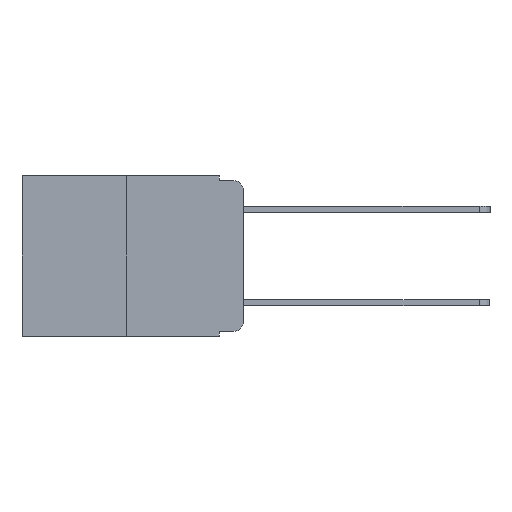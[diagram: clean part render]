
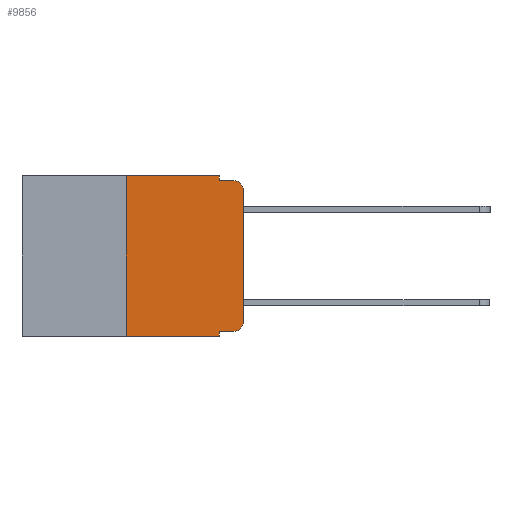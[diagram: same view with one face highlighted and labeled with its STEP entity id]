
A CAD part, left-side view. The second image highlights one B-rep face of the part: STEP entity #9856.
In plain terms, the highlighted planar face has unit normal (-1, 0, 0).
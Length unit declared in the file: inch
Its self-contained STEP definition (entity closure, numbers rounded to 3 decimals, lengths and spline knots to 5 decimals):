
#102 = CIRCLE ( 'NONE', #6710, 0.02 ) ;
#133 = DIRECTION ( 'NONE',  ( -1., 0., 0. ) ) ;
#184 = EDGE_CURVE ( 'NONE', #4571, #2796, #8095, .T. ) ;
#198 = VERTEX_POINT ( 'NONE', #6690 ) ;
#562 = DIRECTION ( 'NONE',  ( 0., -1., 0. ) ) ;
#798 = CARTESIAN_POINT ( 'NONE',  ( 0., 0.25, -0.343 ) ) ;
#813 = ORIENTED_EDGE ( 'NONE', *, *, #11226, .T. ) ;
#899 = VERTEX_POINT ( 'NONE', #11104 ) ;
#1318 = VECTOR ( 'NONE', #3321, 39.37008 ) ;
#1935 = CARTESIAN_POINT ( 'NONE',  ( 0., 0.473, 0. ) ) ;
#1977 = LINE ( 'NONE', #2537, #4477 ) ;
#2357 = CARTESIAN_POINT ( 'NONE',  ( 0., 0., 0. ) ) ;
#2383 = EDGE_CURVE ( 'NONE', #899, #3864, #1977, .T. ) ;
#2537 = CARTESIAN_POINT ( 'NONE',  ( 0., 0.051, -0.333 ) ) ;
#2681 = VERTEX_POINT ( 'NONE', #7798 ) ;
#2796 = VERTEX_POINT ( 'NONE', #7469 ) ;
#2858 = DIRECTION ( 'NONE',  ( 0., 0., -1. ) ) ;
#2948 = CARTESIAN_POINT ( 'NONE',  ( 0., 0.051, -0.343 ) ) ;
#3065 = VERTEX_POINT ( 'NONE', #4823 ) ;
#3231 = DIRECTION ( 'NONE',  ( 0., -1., 0. ) ) ;
#3321 = DIRECTION ( 'NONE',  ( 0., 0., 1. ) ) ;
#3358 = CARTESIAN_POINT ( 'NONE',  ( 0., 0., -0.03 ) ) ;
#3531 = ORIENTED_EDGE ( 'NONE', *, *, #9090, .T. ) ;
#3792 = VECTOR ( 'NONE', #5029, 39.37008 ) ;
#3801 = EDGE_CURVE ( 'NONE', #2796, #198, #11065, .T. ) ;
#3864 = VERTEX_POINT ( 'NONE', #10541 ) ;
#3912 = DIRECTION ( 'NONE',  ( 0., 0., -1. ) ) ;
#3981 = VERTEX_POINT ( 'NONE', #798 ) ;
#4305 = AXIS2_PLACEMENT_3D ( 'NONE', #5704, #133, #6573 ) ;
#4311 = VERTEX_POINT ( 'NONE', #2948 ) ;
#4477 = VECTOR ( 'NONE', #562, 39.37008 ) ;
#4569 = CARTESIAN_POINT ( 'NONE',  ( 0., 0.051, 0. ) ) ;
#4571 = VERTEX_POINT ( 'NONE', #10532 ) ;
#4697 = CIRCLE ( 'NONE', #4305, 0.02 ) ;
#4823 = CARTESIAN_POINT ( 'NONE',  ( 0., 0., -0.313 ) ) ;
#5029 = DIRECTION ( 'NONE',  ( 0., 0., 1. ) ) ;
#5313 = CARTESIAN_POINT ( 'NONE',  ( 0., 0.02, -0.313 ) ) ;
#5469 = AXIS2_PLACEMENT_3D ( 'NONE', #1935, #8231, #2858 ) ;
#5592 = EDGE_CURVE ( 'NONE', #2681, #4571, #10263, .T. ) ;
#5633 = EDGE_LOOP ( 'NONE', ( #9088, #813, #10300, #9795, #8840, #9389, #3531, #9167, #11129, #10483 ) ) ;
#5704 = CARTESIAN_POINT ( 'NONE',  ( 0., 0.02, -0.03 ) ) ;
#5790 = DIRECTION ( 'NONE',  ( 0., -1., 0. ) ) ;
#5833 = VECTOR ( 'NONE', #3912, 39.37008 ) ;
#6018 = CARTESIAN_POINT ( 'NONE',  ( 0., 0.051, 0. ) ) ;
#6226 = DIRECTION ( 'NONE',  ( 0., 0., -1. ) ) ;
#6245 = LINE ( 'NONE', #11028, #3792 ) ;
#6328 = EDGE_CURVE ( 'NONE', #3065, #8122, #6518, .T. ) ;
#6430 = VECTOR ( 'NONE', #7719, 39.37008 ) ;
#6518 = LINE ( 'NONE', #2357, #1318 ) ;
#6573 = DIRECTION ( 'NONE',  ( 0., 0., -1. ) ) ;
#6690 = CARTESIAN_POINT ( 'NONE',  ( 0., 0.02, -0.01 ) ) ;
#6710 = AXIS2_PLACEMENT_3D ( 'NONE', #5313, #11285, #6226 ) ;
#6732 = EDGE_CURVE ( 'NONE', #3981, #2681, #6245, .T. ) ;
#7370 = PLANE ( 'NONE',  #5469 ) ;
#7469 = CARTESIAN_POINT ( 'NONE',  ( 0., 0.051, -0.01 ) ) ;
#7719 = DIRECTION ( 'NONE',  ( 0., 0., -1. ) ) ;
#7749 = FACE_OUTER_BOUND ( 'NONE', #5633, .T. ) ;
#7752 = VECTOR ( 'NONE', #11429, 39.37008 ) ;
#7798 = CARTESIAN_POINT ( 'NONE',  ( 0., 0.25, 0. ) ) ;
#8028 = LINE ( 'NONE', #8894, #7752 ) ;
#8095 = LINE ( 'NONE', #4569, #5833 ) ;
#8122 = VERTEX_POINT ( 'NONE', #3358 ) ;
#8231 = DIRECTION ( 'NONE',  ( 1., 0., 0. ) ) ;
#8681 = LINE ( 'NONE', #6018, #6430 ) ;
#8823 = VECTOR ( 'NONE', #5790, 39.37008 ) ;
#8840 = ORIENTED_EDGE ( 'NONE', *, *, #5592, .F. ) ;
#8894 = CARTESIAN_POINT ( 'NONE',  ( 0., 0.473, -0.343 ) ) ;
#8988 = EDGE_CURVE ( 'NONE', #3864, #3065, #102, .T. ) ;
#9088 = ORIENTED_EDGE ( 'NONE', *, *, #6328, .T. ) ;
#9090 = EDGE_CURVE ( 'NONE', #3981, #4311, #8028, .T. ) ;
#9167 = ORIENTED_EDGE ( 'NONE', *, *, #10335, .F. ) ;
#9389 = ORIENTED_EDGE ( 'NONE', *, *, #6732, .F. ) ;
#9746 = VECTOR ( 'NONE', #3231, 39.37008 ) ;
#9795 = ORIENTED_EDGE ( 'NONE', *, *, #184, .F. ) ;
#9856 = ADVANCED_FACE ( 'NONE', ( #7749 ), #7370, .F. ) ;
#10263 = LINE ( 'NONE', #11253, #9746 ) ;
#10300 = ORIENTED_EDGE ( 'NONE', *, *, #3801, .F. ) ;
#10335 = EDGE_CURVE ( 'NONE', #899, #4311, #8681, .T. ) ;
#10483 = ORIENTED_EDGE ( 'NONE', *, *, #8988, .T. ) ;
#10532 = CARTESIAN_POINT ( 'NONE',  ( 0., 0.051, 0. ) ) ;
#10541 = CARTESIAN_POINT ( 'NONE',  ( 0., 0.02, -0.333 ) ) ;
#11028 = CARTESIAN_POINT ( 'NONE',  ( 0., 0.25, 0. ) ) ;
#11065 = LINE ( 'NONE', #11261, #8823 ) ;
#11104 = CARTESIAN_POINT ( 'NONE',  ( 0., 0.051, -0.333 ) ) ;
#11129 = ORIENTED_EDGE ( 'NONE', *, *, #2383, .T. ) ;
#11226 = EDGE_CURVE ( 'NONE', #8122, #198, #4697, .T. ) ;
#11253 = CARTESIAN_POINT ( 'NONE',  ( 0., 0.473, 0. ) ) ;
#11261 = CARTESIAN_POINT ( 'NONE',  ( 0., 0.051, -0.01 ) ) ;
#11285 = DIRECTION ( 'NONE',  ( -1., 0., 0. ) ) ;
#11429 = DIRECTION ( 'NONE',  ( 0., -1., 0. ) ) ;
